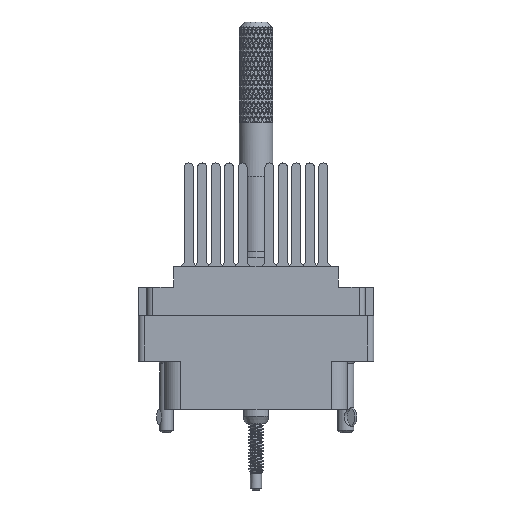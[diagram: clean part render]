
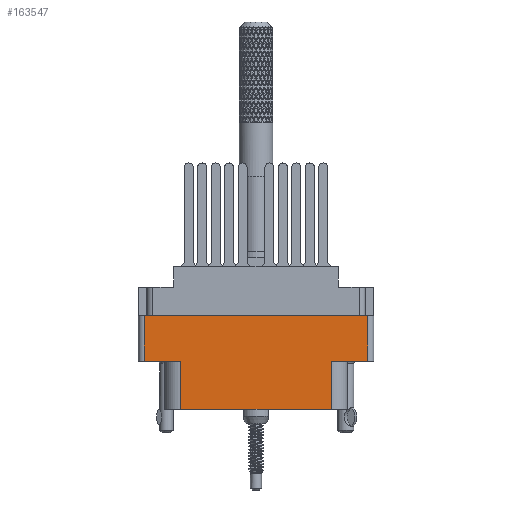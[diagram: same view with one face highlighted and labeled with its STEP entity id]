
A CAD part, front view. The second image highlights one B-rep face of the part: STEP entity #163547.
In plain terms, the highlighted planar face has unit normal (0, -1, 0).
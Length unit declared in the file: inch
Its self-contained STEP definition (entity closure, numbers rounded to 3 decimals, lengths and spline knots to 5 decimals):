
#1900 = CARTESIAN_POINT ( 'NONE',  ( 0., -0.343, -0.529 ) ) ;
#1974 = VERTEX_POINT ( 'NONE', #99665 ) ;
#3296 = ORIENTED_EDGE ( 'NONE', *, *, #194975, .F. ) ;
#3495 = VERTEX_POINT ( 'NONE', #7618 ) ;
#6098 = DIRECTION ( 'NONE',  ( 0., 0., -1. ) ) ;
#7618 = CARTESIAN_POINT ( 'NONE',  ( 0.624, -0.343, -0.274 ) ) ;
#11243 = DIRECTION ( 'NONE',  ( 0., 0., 1. ) ) ;
#14912 = LINE ( 'NONE', #143690, #21978 ) ;
#14951 = ORIENTED_EDGE ( 'NONE', *, *, #159299, .T. ) ;
#17126 = DIRECTION ( 'NONE',  ( -1., 0., 0. ) ) ;
#20839 = CARTESIAN_POINT ( 'NONE',  ( -0.624, -0.343, -0.798 ) ) ;
#21978 = VECTOR ( 'NONE', #160941, 39.37008 ) ;
#24537 = ORIENTED_EDGE ( 'NONE', *, *, #124071, .T. ) ;
#29176 = VERTEX_POINT ( 'NONE', #153326 ) ;
#30781 = VERTEX_POINT ( 'NONE', #55446 ) ;
#34794 = VECTOR ( 'NONE', #79424, 39.37008 ) ;
#36816 = DIRECTION ( 'NONE',  ( 0., 0., -1. ) ) ;
#40007 = LINE ( 'NONE', #1900, #128039 ) ;
#41390 = VECTOR ( 'NONE', #110634, 39.37008 ) ;
#41562 = EDGE_CURVE ( 'NONE', #30781, #101983, #173102, .T. ) ;
#54587 = DIRECTION ( 'NONE',  ( 1., 0., 0. ) ) ;
#55446 = CARTESIAN_POINT ( 'NONE',  ( -0.42052, -0.343, -0.529 ) ) ;
#55829 = EDGE_LOOP ( 'NONE', ( #192547, #24537, #14951, #84870, #102350, #131173, #3296, #112068 ) ) ;
#59954 = FACE_OUTER_BOUND ( 'NONE', #55829, .T. ) ;
#63465 = LINE ( 'NONE', #110020, #34794 ) ;
#65474 = CARTESIAN_POINT ( 'NONE',  ( -0.42052, -0.343, -0.798 ) ) ;
#74885 = VERTEX_POINT ( 'NONE', #194876 ) ;
#79424 = DIRECTION ( 'NONE',  ( 1., 0., 0. ) ) ;
#84870 = ORIENTED_EDGE ( 'NONE', *, *, #41562, .T. ) ;
#92718 = EDGE_CURVE ( 'NONE', #1974, #74885, #154121, .T. ) ;
#94718 = EDGE_CURVE ( 'NONE', #29176, #3495, #63465, .T. ) ;
#99665 = CARTESIAN_POINT ( 'NONE',  ( 0.42052, -0.343, -0.798 ) ) ;
#101983 = VERTEX_POINT ( 'NONE', #137441 ) ;
#102350 = ORIENTED_EDGE ( 'NONE', *, *, #187760, .T. ) ;
#102679 = VECTOR ( 'NONE', #36816, 39.37008 ) ;
#102918 = CARTESIAN_POINT ( 'NONE',  ( 0.42052, -0.343, -0.529 ) ) ;
#110020 = CARTESIAN_POINT ( 'NONE',  ( 0., -0.343, -0.274 ) ) ;
#110128 = VERTEX_POINT ( 'NONE', #148603 ) ;
#110634 = DIRECTION ( 'NONE',  ( 1., 0., 0. ) ) ;
#112068 = ORIENTED_EDGE ( 'NONE', *, *, #154676, .T. ) ;
#114848 = LINE ( 'NONE', #20839, #102679 ) ;
#115803 = AXIS2_PLACEMENT_3D ( 'NONE', #158397, #142413, #6098 ) ;
#124071 = EDGE_CURVE ( 'NONE', #29176, #110128, #114848, .T. ) ;
#124478 = CARTESIAN_POINT ( 'NONE',  ( 0.624, -0.343, -0.529 ) ) ;
#128039 = VECTOR ( 'NONE', #17126, 39.37008 ) ;
#131173 = ORIENTED_EDGE ( 'NONE', *, *, #92718, .T. ) ;
#137441 = CARTESIAN_POINT ( 'NONE',  ( -0.42052, -0.343, -0.798 ) ) ;
#137701 = VECTOR ( 'NONE', #54587, 39.37008 ) ;
#138941 = LINE ( 'NONE', #139916, #41390 ) ;
#139789 = PLANE ( 'NONE',  #115803 ) ;
#139916 = CARTESIAN_POINT ( 'NONE',  ( 0., -0.343, -0.529 ) ) ;
#142413 = DIRECTION ( 'NONE',  ( 0., -1., 0. ) ) ;
#143690 = CARTESIAN_POINT ( 'NONE',  ( 0.624, -0.343, -0.798 ) ) ;
#148603 = CARTESIAN_POINT ( 'NONE',  ( -0.624, -0.343, -0.529 ) ) ;
#153326 = CARTESIAN_POINT ( 'NONE',  ( -0.624, -0.343, -0.274 ) ) ;
#154121 = LINE ( 'NONE', #102918, #175435 ) ;
#154676 = EDGE_CURVE ( 'NONE', #159526, #3495, #14912, .T. ) ;
#158397 = CARTESIAN_POINT ( 'NONE',  ( -0.656, -0.343, -0.798 ) ) ;
#159299 = EDGE_CURVE ( 'NONE', #110128, #30781, #138941, .T. ) ;
#159526 = VERTEX_POINT ( 'NONE', #124478 ) ;
#160941 = DIRECTION ( 'NONE',  ( 0., 0., 1. ) ) ;
#163547 = ADVANCED_FACE ( 'NONE', ( #59954 ), #139789, .T. ) ;
#171852 = DIRECTION ( 'NONE',  ( 0., 0., -1. ) ) ;
#173102 = LINE ( 'NONE', #65474, #187395 ) ;
#175435 = VECTOR ( 'NONE', #11243, 39.37008 ) ;
#178064 = LINE ( 'NONE', #188902, #137701 ) ;
#187395 = VECTOR ( 'NONE', #171852, 39.37008 ) ;
#187760 = EDGE_CURVE ( 'NONE', #101983, #1974, #178064, .T. ) ;
#188902 = CARTESIAN_POINT ( 'NONE',  ( -0.656, -0.343, -0.798 ) ) ;
#192547 = ORIENTED_EDGE ( 'NONE', *, *, #94718, .F. ) ;
#194876 = CARTESIAN_POINT ( 'NONE',  ( 0.42052, -0.343, -0.529 ) ) ;
#194975 = EDGE_CURVE ( 'NONE', #159526, #74885, #40007, .T. ) ;
